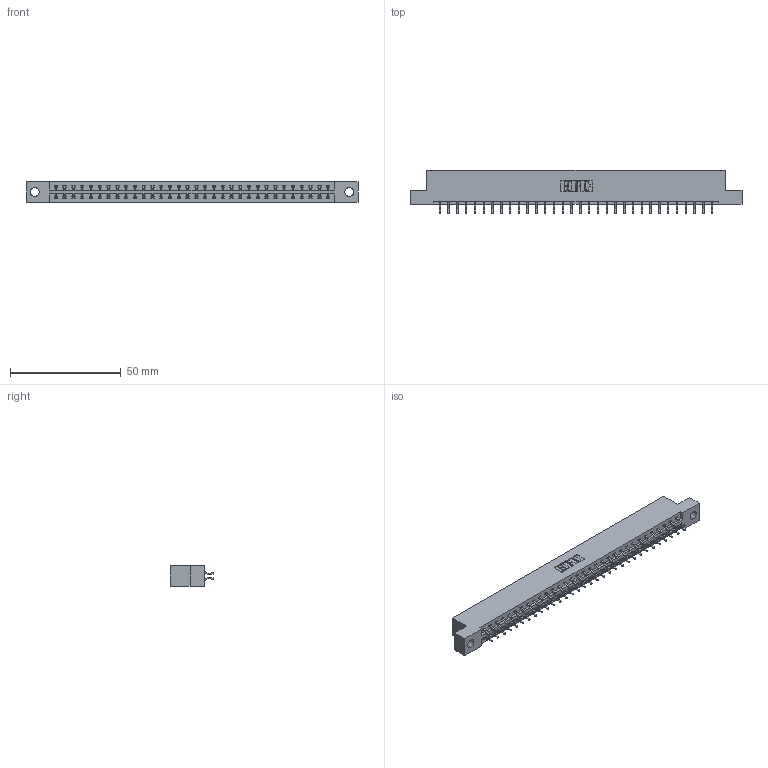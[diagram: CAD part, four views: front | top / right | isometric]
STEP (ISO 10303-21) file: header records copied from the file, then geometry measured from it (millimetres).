
FILE_DESCRIPTION (( 'STEP AP203' ), '1' );
FILE_NAME ('337-064-556-204.STEP', '2019-10-09T22:31:37', ( '' ), ( '' ), 'SwSTEP 2.0', 'SolidWorks 2016', '' );
FILE_SCHEMA (( 'CONFIG_CONTROL_DESIGN' ));
Length unit declared in the file: inch
Products named in the file (3): 337-064-556-204; 337 Part_Flush Mounting Lugs - 0.156 Dia-TH; 345-292-001_556 Tail
Assembly tree (65 placements, depth 2):
  337-064-556-204
    337 Part_Flush Mounting Lugs - 0.156 Dia-TH
    345-292-001_556 Tail  x64
Bounding box: 149.81 x 19.57 x 9.4 mm (x, y, z)
Volume: 15564.6 mm3; surface area: 17228.5 mm2
Topology: 65 solids, 65 shells, 3954 faces, 11767 edges, 7758 vertices
Faces by surface type: plane 2758, cylinder 1196
Entity records: 26327 total; most frequent: CARTESIAN_POINT 4458, ORIENTED_EDGE 4382, DIRECTION 3799, EDGE_CURVE 2191, LINE 2055, VECTOR 2055, VERTEX_POINT 1458, AXIS2_PLACEMENT_3D 872
